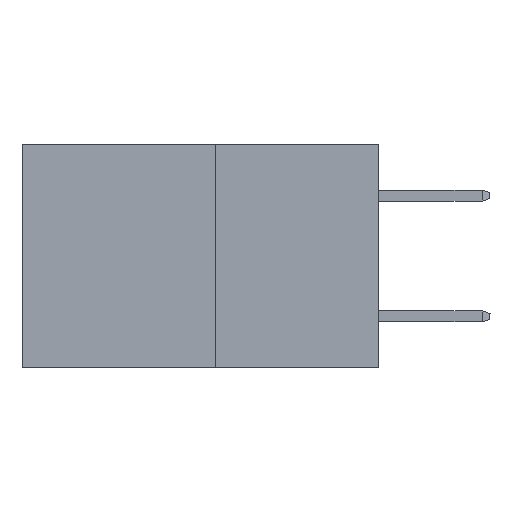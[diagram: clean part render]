
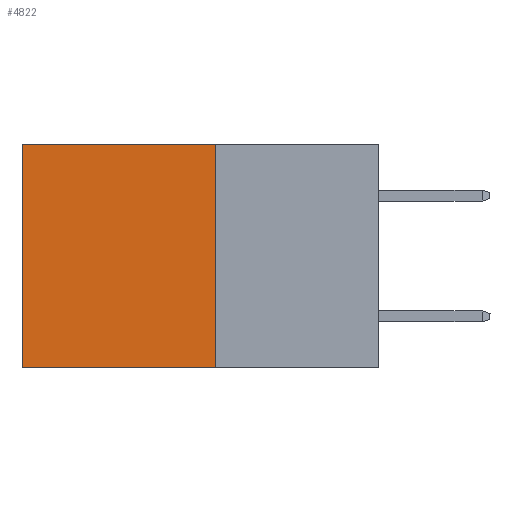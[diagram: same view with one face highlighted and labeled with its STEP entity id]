
A CAD part, left-side view. The second image highlights one B-rep face of the part: STEP entity #4822.
In plain terms, the highlighted planar face has unit normal (-1, 0, 0).
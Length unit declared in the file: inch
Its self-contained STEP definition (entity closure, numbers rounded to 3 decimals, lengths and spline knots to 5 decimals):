
#360 = CARTESIAN_POINT ( 'NONE',  ( 0.277, 0.27, -0.37 ) ) ;
#1502 = DIRECTION ( 'NONE',  ( 0., 0., -1. ) ) ;
#3274 = LINE ( 'NONE', #10096, #15641 ) ;
#3359 = VECTOR ( 'NONE', #19063, 39.37008 ) ;
#4051 = CARTESIAN_POINT ( 'NONE',  ( 0.277, 0.59, -0.37 ) ) ;
#4604 = CARTESIAN_POINT ( 'NONE',  ( 0.277, 0.59, -0.37 ) ) ;
#4822 = ADVANCED_FACE ( 'NONE', ( #15744 ), #5460, .F. ) ;
#5219 = EDGE_CURVE ( 'NONE', #16068, #23047, #22931, .T. ) ;
#5460 = PLANE ( 'NONE',  #29661 ) ;
#6500 = VERTEX_POINT ( 'NONE', #21075 ) ;
#7996 = DIRECTION ( 'NONE',  ( 1., 0., 0. ) ) ;
#10096 = CARTESIAN_POINT ( 'NONE',  ( 0.277, 0.27, -0.37 ) ) ;
#11335 = EDGE_CURVE ( 'NONE', #17241, #6500, #25288, .T. ) ;
#12518 = DIRECTION ( 'NONE',  ( 0., 0., -1. ) ) ;
#14288 = EDGE_CURVE ( 'NONE', #17241, #16068, #3274, .T. ) ;
#14496 = CARTESIAN_POINT ( 'NONE',  ( 0.277, 0.27, -0.37 ) ) ;
#15166 = ORIENTED_EDGE ( 'NONE', *, *, #24975, .T. ) ;
#15335 = LINE ( 'NONE', #4051, #26713 ) ;
#15641 = VECTOR ( 'NONE', #12518, 39.37008 ) ;
#15744 = FACE_OUTER_BOUND ( 'NONE', #24119, .T. ) ;
#16068 = VERTEX_POINT ( 'NONE', #14496 ) ;
#16521 = CARTESIAN_POINT ( 'NONE',  ( 0.277, 0.27, 0. ) ) ;
#16606 = CARTESIAN_POINT ( 'NONE',  ( 0.277, 0.27, -0.37 ) ) ;
#17175 = ORIENTED_EDGE ( 'NONE', *, *, #14288, .F. ) ;
#17241 = VERTEX_POINT ( 'NONE', #16521 ) ;
#17483 = ORIENTED_EDGE ( 'NONE', *, *, #5219, .F. ) ;
#19063 = DIRECTION ( 'NONE',  ( 0., 1., 0. ) ) ;
#19864 = ORIENTED_EDGE ( 'NONE', *, *, #11335, .T. ) ;
#21075 = CARTESIAN_POINT ( 'NONE',  ( 0.277, 0.59, 0. ) ) ;
#22931 = LINE ( 'NONE', #16606, #3359 ) ;
#23047 = VERTEX_POINT ( 'NONE', #4604 ) ;
#24119 = EDGE_LOOP ( 'NONE', ( #15166, #17483, #17175, #19864 ) ) ;
#24535 = VECTOR ( 'NONE', #29341, 39.37008 ) ;
#24975 = EDGE_CURVE ( 'NONE', #6500, #23047, #15335, .T. ) ;
#25021 = DIRECTION ( 'NONE',  ( 0., 0., -1. ) ) ;
#25288 = LINE ( 'NONE', #26927, #24535 ) ;
#26713 = VECTOR ( 'NONE', #1502, 39.37008 ) ;
#26927 = CARTESIAN_POINT ( 'NONE',  ( 0.277, 0.27, 0. ) ) ;
#29341 = DIRECTION ( 'NONE',  ( 0., 1., 0. ) ) ;
#29661 = AXIS2_PLACEMENT_3D ( 'NONE', #360, #7996, #25021 ) ;
